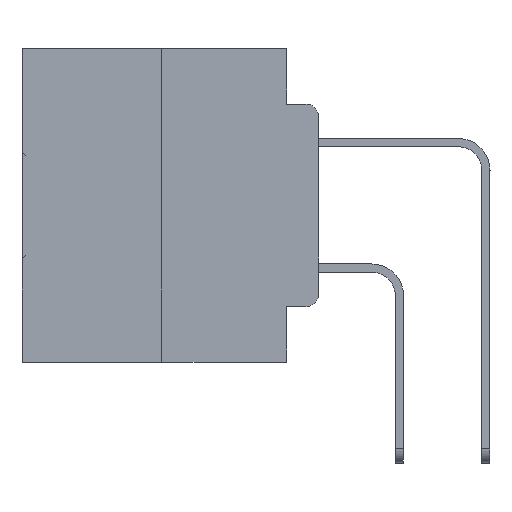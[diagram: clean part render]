
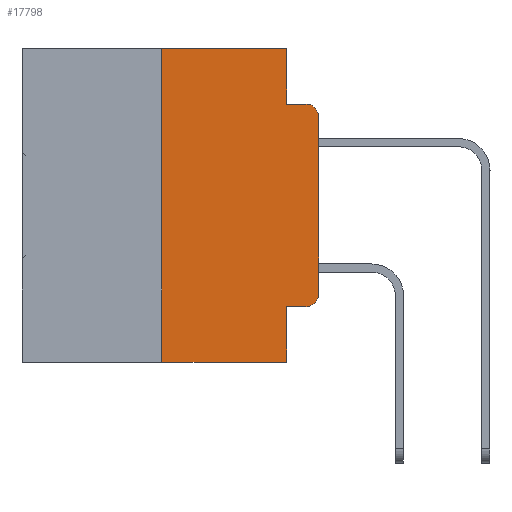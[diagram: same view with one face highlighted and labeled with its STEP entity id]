
A CAD part, left-side view. The second image highlights one B-rep face of the part: STEP entity #17798.
In plain terms, the highlighted planar face has unit normal (-1, 0, 0).
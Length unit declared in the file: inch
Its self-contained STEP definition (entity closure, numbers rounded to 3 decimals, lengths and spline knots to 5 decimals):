
#10 = CIRCLE ( 'NONE', #25986, 0.02 ) ;
#245 = VERTEX_POINT ( 'NONE', #17529 ) ;
#348 = LINE ( 'NONE', #32041, #23659 ) ;
#1189 = ORIENTED_EDGE ( 'NONE', *, *, #17851, .F. ) ;
#1811 = CARTESIAN_POINT ( 'NONE',  ( 0., 0.25, -0.5 ) ) ;
#2252 = DIRECTION ( 'NONE',  ( 1., 0., 0. ) ) ;
#2592 = CARTESIAN_POINT ( 'NONE',  ( 0., 0.473, 0. ) ) ;
#3280 = CARTESIAN_POINT ( 'NONE',  ( 0., 0.051, -0.0885 ) ) ;
#5117 = ORIENTED_EDGE ( 'NONE', *, *, #34077, .F. ) ;
#5746 = CARTESIAN_POINT ( 'NONE',  ( 0., 0.02, -0.3915 ) ) ;
#6345 = VERTEX_POINT ( 'NONE', #24316 ) ;
#6726 = VECTOR ( 'NONE', #17979, 39.37008 ) ;
#6784 = EDGE_CURVE ( 'NONE', #33222, #16537, #30187, .T. ) ;
#6861 = EDGE_CURVE ( 'NONE', #8380, #32510, #22352, .T. ) ;
#6950 = LINE ( 'NONE', #30498, #15889 ) ;
#7094 = ORIENTED_EDGE ( 'NONE', *, *, #18672, .F. ) ;
#7593 = CARTESIAN_POINT ( 'NONE',  ( 0., 0.02, -0.1085 ) ) ;
#7994 = LINE ( 'NONE', #3280, #24133 ) ;
#8187 = DIRECTION ( 'NONE',  ( 0., 0., -1. ) ) ;
#8380 = VERTEX_POINT ( 'NONE', #12857 ) ;
#8634 = VECTOR ( 'NONE', #24161, 39.37008 ) ;
#9112 = ORIENTED_EDGE ( 'NONE', *, *, #6861, .F. ) ;
#9696 = VECTOR ( 'NONE', #27187, 39.37008 ) ;
#10511 = EDGE_CURVE ( 'NONE', #16537, #30213, #348, .T. ) ;
#10623 = CARTESIAN_POINT ( 'NONE',  ( 0., 0.02, -0.4115 ) ) ;
#10739 = ORIENTED_EDGE ( 'NONE', *, *, #12912, .T. ) ;
#11493 = VECTOR ( 'NONE', #29401, 39.37008 ) ;
#12350 = VERTEX_POINT ( 'NONE', #16299 ) ;
#12857 = CARTESIAN_POINT ( 'NONE',  ( 0., 0.051, 0. ) ) ;
#12912 = EDGE_CURVE ( 'NONE', #30213, #245, #10, .T. ) ;
#13131 = CARTESIAN_POINT ( 'NONE',  ( 0., 0.051, -0.4115 ) ) ;
#13734 = EDGE_LOOP ( 'NONE', ( #33570, #10739, #1189, #9112, #28808, #7094, #22428, #5117, #28670, #21392 ) ) ;
#15889 = VECTOR ( 'NONE', #19621, 39.37008 ) ;
#16299 = CARTESIAN_POINT ( 'NONE',  ( 0., 0.051, -0.5 ) ) ;
#16537 = VERTEX_POINT ( 'NONE', #33907 ) ;
#16616 = CARTESIAN_POINT ( 'NONE',  ( 0., 0.051, -0.0885 ) ) ;
#16622 = LINE ( 'NONE', #18882, #11493 ) ;
#17074 = EDGE_CURVE ( 'NONE', #22011, #12350, #27250, .T. ) ;
#17176 = VECTOR ( 'NONE', #23670, 39.37008 ) ;
#17529 = CARTESIAN_POINT ( 'NONE',  ( 0., 0.02, -0.0885 ) ) ;
#17605 = EDGE_CURVE ( 'NONE', #6345, #8380, #6950, .T. ) ;
#17798 = ADVANCED_FACE ( 'NONE', ( #33781 ), #17883, .F. ) ;
#17851 = EDGE_CURVE ( 'NONE', #32510, #245, #7994, .T. ) ;
#17883 = PLANE ( 'NONE',  #29666 ) ;
#17979 = DIRECTION ( 'NONE',  ( 0., 0., -1. ) ) ;
#18166 = DIRECTION ( 'NONE',  ( -1., 0., 0. ) ) ;
#18491 = CARTESIAN_POINT ( 'NONE',  ( 0., 0.051, 0. ) ) ;
#18672 = EDGE_CURVE ( 'NONE', #22011, #6345, #16622, .T. ) ;
#18882 = CARTESIAN_POINT ( 'NONE',  ( 0., 0.25, 0. ) ) ;
#18926 = DIRECTION ( 'NONE',  ( 0., 0., 1. ) ) ;
#19621 = DIRECTION ( 'NONE',  ( 0., -1., 0. ) ) ;
#20641 = DIRECTION ( 'NONE',  ( 0., 0., -1. ) ) ;
#21392 = ORIENTED_EDGE ( 'NONE', *, *, #6784, .T. ) ;
#22011 = VERTEX_POINT ( 'NONE', #1811 ) ;
#22352 = LINE ( 'NONE', #22520, #9696 ) ;
#22428 = ORIENTED_EDGE ( 'NONE', *, *, #17074, .T. ) ;
#22520 = CARTESIAN_POINT ( 'NONE',  ( 0., 0.051, 0. ) ) ;
#22725 = CARTESIAN_POINT ( 'NONE',  ( 0., 0.051, -0.4115 ) ) ;
#23286 = EDGE_CURVE ( 'NONE', #31744, #33222, #23846, .T. ) ;
#23659 = VECTOR ( 'NONE', #18926, 39.37008 ) ;
#23670 = DIRECTION ( 'NONE',  ( 0., -1., 0. ) ) ;
#23846 = LINE ( 'NONE', #13131, #17176 ) ;
#24133 = VECTOR ( 'NONE', #24424, 39.37008 ) ;
#24161 = DIRECTION ( 'NONE',  ( 0., -1., 0. ) ) ;
#24316 = CARTESIAN_POINT ( 'NONE',  ( 0., 0.25, 0. ) ) ;
#24424 = DIRECTION ( 'NONE',  ( 0., -1., 0. ) ) ;
#24674 = CARTESIAN_POINT ( 'NONE',  ( 0., 0.473, -0.5 ) ) ;
#25320 = CARTESIAN_POINT ( 'NONE',  ( 0., 0., -0.1085 ) ) ;
#25986 = AXIS2_PLACEMENT_3D ( 'NONE', #7593, #18166, #28689 ) ;
#26511 = DIRECTION ( 'NONE',  ( -1., 0., 0. ) ) ;
#27187 = DIRECTION ( 'NONE',  ( 0., 0., -1. ) ) ;
#27250 = LINE ( 'NONE', #24674, #8634 ) ;
#28670 = ORIENTED_EDGE ( 'NONE', *, *, #23286, .T. ) ;
#28689 = DIRECTION ( 'NONE',  ( 0., 0., -1. ) ) ;
#28808 = ORIENTED_EDGE ( 'NONE', *, *, #17605, .F. ) ;
#29401 = DIRECTION ( 'NONE',  ( 0., 0., 1. ) ) ;
#29666 = AXIS2_PLACEMENT_3D ( 'NONE', #2592, #2252, #20641 ) ;
#30187 = CIRCLE ( 'NONE', #33487, 0.02 ) ;
#30213 = VERTEX_POINT ( 'NONE', #25320 ) ;
#30498 = CARTESIAN_POINT ( 'NONE',  ( 0., 0.473, 0. ) ) ;
#31744 = VERTEX_POINT ( 'NONE', #22725 ) ;
#32041 = CARTESIAN_POINT ( 'NONE',  ( 0., 0., 0. ) ) ;
#32510 = VERTEX_POINT ( 'NONE', #16616 ) ;
#33222 = VERTEX_POINT ( 'NONE', #10623 ) ;
#33487 = AXIS2_PLACEMENT_3D ( 'NONE', #5746, #26511, #8187 ) ;
#33570 = ORIENTED_EDGE ( 'NONE', *, *, #10511, .T. ) ;
#33781 = FACE_OUTER_BOUND ( 'NONE', #13734, .T. ) ;
#33907 = CARTESIAN_POINT ( 'NONE',  ( 0., 0., -0.3915 ) ) ;
#34077 = EDGE_CURVE ( 'NONE', #31744, #12350, #34218, .T. ) ;
#34218 = LINE ( 'NONE', #18491, #6726 ) ;
